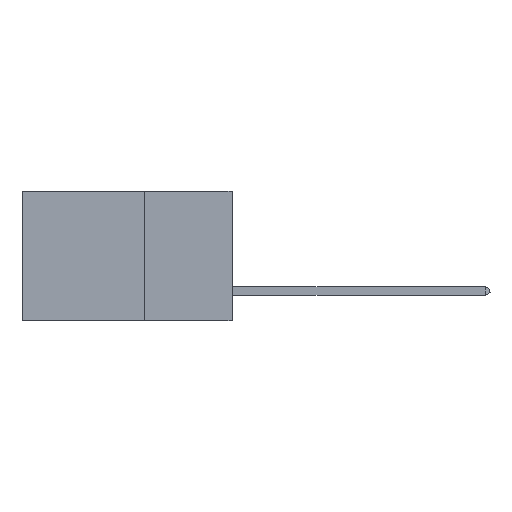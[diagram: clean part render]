
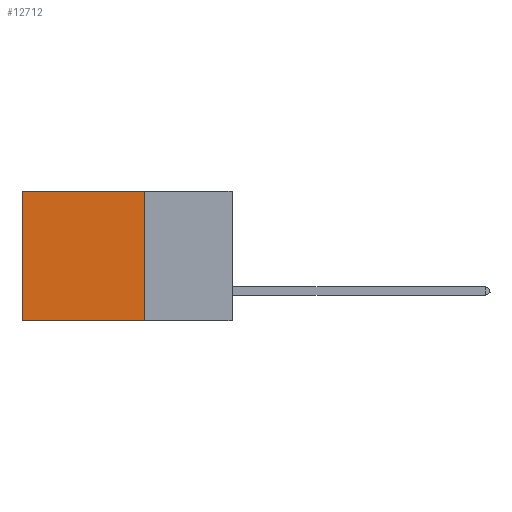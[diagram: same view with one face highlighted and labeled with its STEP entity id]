
A CAD part, left-side view. The second image highlights one B-rep face of the part: STEP entity #12712.
In plain terms, the highlighted planar face has unit normal (-1, 0, 0).
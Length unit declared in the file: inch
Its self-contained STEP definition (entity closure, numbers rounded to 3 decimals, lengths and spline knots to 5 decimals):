
#64 = LINE ( 'NONE', #13997, #10638 ) ;
#1173 = VECTOR ( 'NONE', #15801, 39.37008 ) ;
#2634 = CARTESIAN_POINT ( 'NONE',  ( 0.2875, 0.25, 0. ) ) ;
#3738 = ORIENTED_EDGE ( 'NONE', *, *, #8322, .F. ) ;
#4799 = LINE ( 'NONE', #2634, #1173 ) ;
#4863 = EDGE_CURVE ( 'NONE', #27163, #21622, #19167, .T. ) ;
#6352 = DIRECTION ( 'NONE',  ( 1., 0., 0. ) ) ;
#7269 = CARTESIAN_POINT ( 'NONE',  ( 0.2875, 0.6, -0.37 ) ) ;
#7573 = LINE ( 'NONE', #14745, #8563 ) ;
#8322 = EDGE_CURVE ( 'NONE', #11275, #21622, #7573, .T. ) ;
#8563 = VECTOR ( 'NONE', #18692, 39.37008 ) ;
#8659 = CARTESIAN_POINT ( 'NONE',  ( 0.2875, 0.25, 0. ) ) ;
#9539 = CARTESIAN_POINT ( 'NONE',  ( 0.2875, 0.6, 0. ) ) ;
#9843 = EDGE_CURVE ( 'NONE', #14779, #11275, #4799, .T. ) ;
#10606 = PLANE ( 'NONE',  #18808 ) ;
#10638 = VECTOR ( 'NONE', #20459, 39.37008 ) ;
#11275 = VERTEX_POINT ( 'NONE', #20410 ) ;
#12712 = ADVANCED_FACE ( 'NONE', ( #16905 ), #10606, .F. ) ;
#13996 = CARTESIAN_POINT ( 'NONE',  ( 0.2875, 0.25, 0. ) ) ;
#13997 = CARTESIAN_POINT ( 'NONE',  ( 0.2875, 0.25, 0. ) ) ;
#14745 = CARTESIAN_POINT ( 'NONE',  ( 0.2875, 0.25, -0.37 ) ) ;
#14779 = VERTEX_POINT ( 'NONE', #13996 ) ;
#15078 = ORIENTED_EDGE ( 'NONE', *, *, #4863, .T. ) ;
#15220 = CARTESIAN_POINT ( 'NONE',  ( 0.2875, 0.6, 0. ) ) ;
#15801 = DIRECTION ( 'NONE',  ( 0., 0., -1. ) ) ;
#16905 = FACE_OUTER_BOUND ( 'NONE', #24999, .T. ) ;
#18169 = EDGE_CURVE ( 'NONE', #14779, #27163, #64, .T. ) ;
#18692 = DIRECTION ( 'NONE',  ( 0., 1., 0. ) ) ;
#18808 = AXIS2_PLACEMENT_3D ( 'NONE', #8659, #6352, #25524 ) ;
#19167 = LINE ( 'NONE', #9539, #22462 ) ;
#20410 = CARTESIAN_POINT ( 'NONE',  ( 0.2875, 0.25, -0.37 ) ) ;
#20459 = DIRECTION ( 'NONE',  ( 0., 1., 0. ) ) ;
#21622 = VERTEX_POINT ( 'NONE', #7269 ) ;
#22462 = VECTOR ( 'NONE', #24005, 39.37008 ) ;
#23340 = ORIENTED_EDGE ( 'NONE', *, *, #9843, .F. ) ;
#24005 = DIRECTION ( 'NONE',  ( 0., 0., -1. ) ) ;
#24999 = EDGE_LOOP ( 'NONE', ( #15078, #3738, #23340, #26468 ) ) ;
#25524 = DIRECTION ( 'NONE',  ( 0., 0., -1. ) ) ;
#26468 = ORIENTED_EDGE ( 'NONE', *, *, #18169, .T. ) ;
#27163 = VERTEX_POINT ( 'NONE', #15220 ) ;
